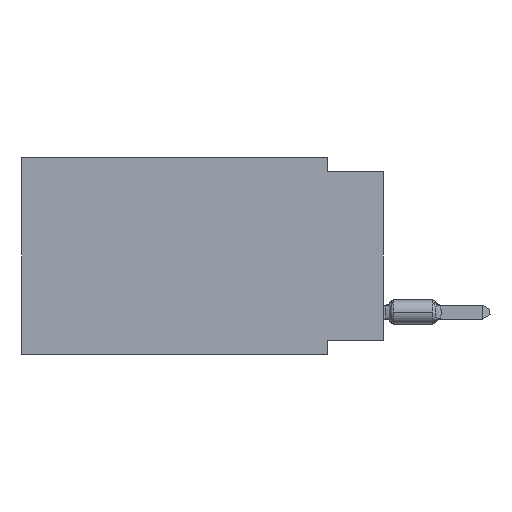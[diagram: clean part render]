
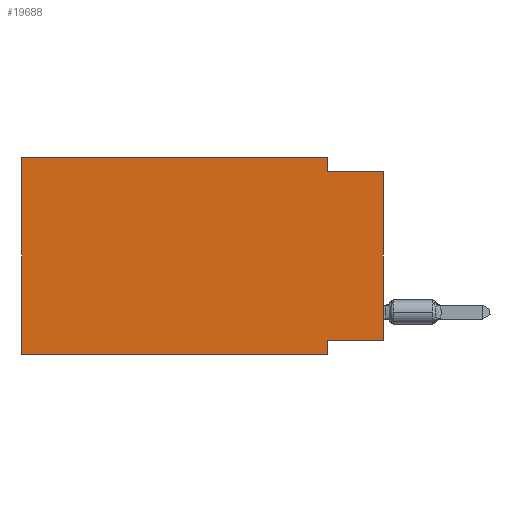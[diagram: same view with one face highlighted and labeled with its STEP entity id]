
A CAD part, left-side view. The second image highlights one B-rep face of the part: STEP entity #19688.
In plain terms, the highlighted planar face has unit normal (-1, 0, 0).
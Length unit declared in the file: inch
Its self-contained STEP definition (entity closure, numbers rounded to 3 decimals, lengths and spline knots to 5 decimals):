
#930 = EDGE_CURVE ( 'NONE', #44028, #20248, #31715, .T. ) ;
#958 = DIRECTION ( 'NONE',  ( 0., -1., 0. ) ) ;
#969 = LINE ( 'NONE', #34661, #40941 ) ;
#1090 = CARTESIAN_POINT ( 'NONE',  ( 0., 0.645, 0. ) ) ;
#2333 = ORIENTED_EDGE ( 'NONE', *, *, #40183, .F. ) ;
#3083 = VECTOR ( 'NONE', #30838, 39.37008 ) ;
#3799 = ORIENTED_EDGE ( 'NONE', *, *, #12867, .F. ) ;
#4100 = DIRECTION ( 'NONE',  ( 0., 0., -1. ) ) ;
#4246 = VECTOR ( 'NONE', #28546, 39.37008 ) ;
#4337 = CARTESIAN_POINT ( 'NONE',  ( 0., 0., -0.025 ) ) ;
#5892 = LINE ( 'NONE', #29899, #24992 ) ;
#7926 = EDGE_CURVE ( 'NONE', #40663, #31028, #38043, .T. ) ;
#8573 = VERTEX_POINT ( 'NONE', #35928 ) ;
#10206 = EDGE_LOOP ( 'NONE', ( #41020, #2333, #3799, #39895, #40697, #19959, #43480, #23192 ) ) ;
#12827 = EDGE_CURVE ( 'NONE', #44028, #8573, #18673, .T. ) ;
#12867 = EDGE_CURVE ( 'NONE', #27540, #15339, #42250, .T. ) ;
#13345 = VECTOR ( 'NONE', #958, 39.37008 ) ;
#13969 = EDGE_CURVE ( 'NONE', #31028, #20248, #36272, .T. ) ;
#14851 = VERTEX_POINT ( 'NONE', #4337 ) ;
#15339 = VERTEX_POINT ( 'NONE', #33365 ) ;
#15397 = DIRECTION ( 'NONE',  ( 0., -1., 0. ) ) ;
#18152 = FACE_OUTER_BOUND ( 'NONE', #10206, .T. ) ;
#18452 = CARTESIAN_POINT ( 'NONE',  ( 0., 0.1, 0. ) ) ;
#18673 = LINE ( 'NONE', #22033, #4246 ) ;
#18885 = EDGE_CURVE ( 'NONE', #8573, #27540, #969, .T. ) ;
#19688 = ADVANCED_FACE ( 'NONE', ( #18152 ), #31847, .F. ) ;
#19883 = VECTOR ( 'NONE', #43225, 39.37008 ) ;
#19959 = ORIENTED_EDGE ( 'NONE', *, *, #930, .T. ) ;
#20248 = VERTEX_POINT ( 'NONE', #37606 ) ;
#21285 = CARTESIAN_POINT ( 'NONE',  ( 0., 0., -0.325 ) ) ;
#21477 = VECTOR ( 'NONE', #4100, 39.37008 ) ;
#21590 = CARTESIAN_POINT ( 'NONE',  ( 0., 0.1, 0. ) ) ;
#21701 = CARTESIAN_POINT ( 'NONE',  ( 0., 0.1, -0.35 ) ) ;
#22033 = CARTESIAN_POINT ( 'NONE',  ( 0., 0.645, 0. ) ) ;
#22571 = LINE ( 'NONE', #40094, #39872 ) ;
#23192 = ORIENTED_EDGE ( 'NONE', *, *, #7926, .F. ) ;
#23890 = CARTESIAN_POINT ( 'NONE',  ( 0., 0., -0.325 ) ) ;
#24992 = VECTOR ( 'NONE', #43820, 39.37008 ) ;
#25102 = DIRECTION ( 'NONE',  ( 1., 0., 0. ) ) ;
#26546 = EDGE_CURVE ( 'NONE', #40663, #14851, #5892, .T. ) ;
#27540 = VERTEX_POINT ( 'NONE', #21590 ) ;
#27917 = CARTESIAN_POINT ( 'NONE',  ( 0., 0.645, -0.35 ) ) ;
#28053 = CARTESIAN_POINT ( 'NONE',  ( 0., 0.1, -0.325 ) ) ;
#28546 = DIRECTION ( 'NONE',  ( 0., 0., 1. ) ) ;
#28785 = CARTESIAN_POINT ( 'NONE',  ( 0., 0.645, -0.35 ) ) ;
#29899 = CARTESIAN_POINT ( 'NONE',  ( 0., 0., 0. ) ) ;
#30838 = DIRECTION ( 'NONE',  ( 0., 1., 0. ) ) ;
#31028 = VERTEX_POINT ( 'NONE', #28053 ) ;
#31715 = LINE ( 'NONE', #28785, #13345 ) ;
#31847 = PLANE ( 'NONE',  #33847 ) ;
#33365 = CARTESIAN_POINT ( 'NONE',  ( 0., 0.1, -0.025 ) ) ;
#33847 = AXIS2_PLACEMENT_3D ( 'NONE', #1090, #25102, #38822 ) ;
#34661 = CARTESIAN_POINT ( 'NONE',  ( 0., 0.645, 0. ) ) ;
#35114 = DIRECTION ( 'NONE',  ( 0., -1., 0. ) ) ;
#35928 = CARTESIAN_POINT ( 'NONE',  ( 0., 0.645, 0. ) ) ;
#36272 = LINE ( 'NONE', #21701, #19883 ) ;
#37606 = CARTESIAN_POINT ( 'NONE',  ( 0., 0.1, -0.35 ) ) ;
#38043 = LINE ( 'NONE', #23890, #3083 ) ;
#38822 = DIRECTION ( 'NONE',  ( 0., 0., -1. ) ) ;
#39872 = VECTOR ( 'NONE', #15397, 39.37008 ) ;
#39895 = ORIENTED_EDGE ( 'NONE', *, *, #18885, .F. ) ;
#40094 = CARTESIAN_POINT ( 'NONE',  ( 0., 0., -0.025 ) ) ;
#40183 = EDGE_CURVE ( 'NONE', #15339, #14851, #22571, .T. ) ;
#40663 = VERTEX_POINT ( 'NONE', #21285 ) ;
#40697 = ORIENTED_EDGE ( 'NONE', *, *, #12827, .F. ) ;
#40941 = VECTOR ( 'NONE', #35114, 39.37008 ) ;
#41020 = ORIENTED_EDGE ( 'NONE', *, *, #26546, .T. ) ;
#42250 = LINE ( 'NONE', #18452, #21477 ) ;
#43225 = DIRECTION ( 'NONE',  ( 0., 0., -1. ) ) ;
#43480 = ORIENTED_EDGE ( 'NONE', *, *, #13969, .F. ) ;
#43820 = DIRECTION ( 'NONE',  ( 0., 0., 1. ) ) ;
#44028 = VERTEX_POINT ( 'NONE', #27917 ) ;
